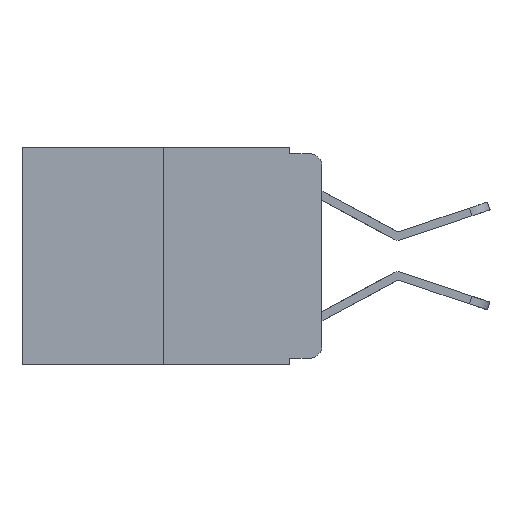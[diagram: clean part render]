
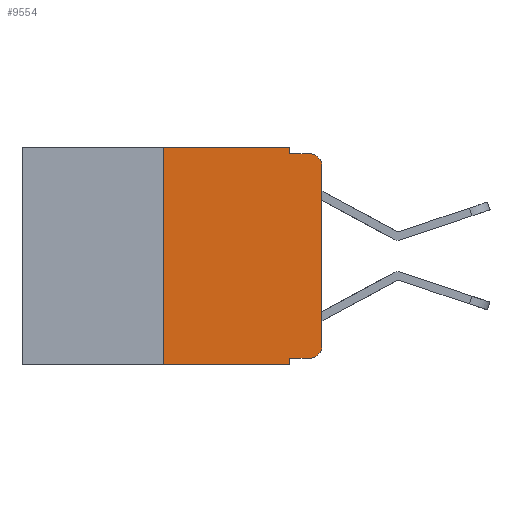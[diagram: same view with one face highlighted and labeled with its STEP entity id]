
A CAD part, left-side view. The second image highlights one B-rep face of the part: STEP entity #9554.
In plain terms, the highlighted planar face has unit normal (-1, 0, 0).
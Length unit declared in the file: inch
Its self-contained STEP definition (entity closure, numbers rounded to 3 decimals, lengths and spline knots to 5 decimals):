
#33 = CARTESIAN_POINT ( 'NONE',  ( 0., 0.473, 0. ) ) ;
#319 = CARTESIAN_POINT ( 'NONE',  ( 0., 0., 0. ) ) ;
#539 = DIRECTION ( 'NONE',  ( -1., 0., 0. ) ) ;
#790 = VECTOR ( 'NONE', #9614, 39.37008 ) ;
#947 = LINE ( 'NONE', #33, #13741 ) ;
#1215 = LINE ( 'NONE', #3589, #790 ) ;
#1332 = FACE_OUTER_BOUND ( 'NONE', #8569, .T. ) ;
#1608 = VERTEX_POINT ( 'NONE', #3708 ) ;
#1695 = ORIENTED_EDGE ( 'NONE', *, *, #7342, .F. ) ;
#1735 = AXIS2_PLACEMENT_3D ( 'NONE', #8056, #539, #9251 ) ;
#2065 = LINE ( 'NONE', #319, #2474 ) ;
#2474 = VECTOR ( 'NONE', #9069, 39.37008 ) ;
#2767 = DIRECTION ( 'NONE',  ( 0., -1., 0. ) ) ;
#2843 = DIRECTION ( 'NONE',  ( 0., -1., 0. ) ) ;
#2964 = ORIENTED_EDGE ( 'NONE', *, *, #14952, .T. ) ;
#3030 = VERTEX_POINT ( 'NONE', #7728 ) ;
#3143 = ORIENTED_EDGE ( 'NONE', *, *, #15994, .F. ) ;
#3589 = CARTESIAN_POINT ( 'NONE',  ( 0., 0.051, 0. ) ) ;
#3666 = PLANE ( 'NONE',  #10680 ) ;
#3708 = CARTESIAN_POINT ( 'NONE',  ( 0., 0., -0.03 ) ) ;
#3801 = ORIENTED_EDGE ( 'NONE', *, *, #5051, .F. ) ;
#4119 = DIRECTION ( 'NONE',  ( 0., -1., 0. ) ) ;
#4185 = DIRECTION ( 'NONE',  ( 0., 0., 1. ) ) ;
#4204 = VERTEX_POINT ( 'NONE', #11322 ) ;
#4241 = VERTEX_POINT ( 'NONE', #11829 ) ;
#4921 = DIRECTION ( 'NONE',  ( 0., 0., -1. ) ) ;
#4965 = ORIENTED_EDGE ( 'NONE', *, *, #9087, .T. ) ;
#5051 = EDGE_CURVE ( 'NONE', #4241, #13048, #6889, .T. ) ;
#5400 = VERTEX_POINT ( 'NONE', #9949 ) ;
#5528 = CARTESIAN_POINT ( 'NONE',  ( 0., 0., -0.313 ) ) ;
#6500 = CARTESIAN_POINT ( 'NONE',  ( 0., 0.02, -0.03 ) ) ;
#6889 = LINE ( 'NONE', #6901, #9726 ) ;
#6901 = CARTESIAN_POINT ( 'NONE',  ( 0., 0.051, 0. ) ) ;
#7060 = CARTESIAN_POINT ( 'NONE',  ( 0., 0.473, 0. ) ) ;
#7342 = EDGE_CURVE ( 'NONE', #4204, #11573, #947, .T. ) ;
#7368 = EDGE_CURVE ( 'NONE', #1608, #15202, #10515, .T. ) ;
#7493 = VERTEX_POINT ( 'NONE', #5528 ) ;
#7577 = VECTOR ( 'NONE', #12382, 39.37008 ) ;
#7620 = CARTESIAN_POINT ( 'NONE',  ( 0., 0.051, -0.01 ) ) ;
#7711 = DIRECTION ( 'NONE',  ( 0., 0., -1. ) ) ;
#7728 = CARTESIAN_POINT ( 'NONE',  ( 0., 0.25, -0.343 ) ) ;
#7968 = LINE ( 'NONE', #9928, #7577 ) ;
#8056 = CARTESIAN_POINT ( 'NONE',  ( 0., 0.02, -0.313 ) ) ;
#8528 = ORIENTED_EDGE ( 'NONE', *, *, #9886, .T. ) ;
#8569 = EDGE_LOOP ( 'NONE', ( #9623, #10857, #14451, #3143, #1695, #9246, #2964, #3801, #4965, #8528 ) ) ;
#8946 = CARTESIAN_POINT ( 'NONE',  ( 0., 0.051, -0.01 ) ) ;
#8979 = CARTESIAN_POINT ( 'NONE',  ( 0., 0.25, 0. ) ) ;
#9069 = DIRECTION ( 'NONE',  ( 0., 0., 1. ) ) ;
#9087 = EDGE_CURVE ( 'NONE', #4241, #5400, #7968, .T. ) ;
#9246 = ORIENTED_EDGE ( 'NONE', *, *, #12351, .F. ) ;
#9251 = DIRECTION ( 'NONE',  ( 0., 0., -1. ) ) ;
#9341 = VECTOR ( 'NONE', #4185, 39.37008 ) ;
#9554 = ADVANCED_FACE ( 'NONE', ( #1332 ), #3666, .F. ) ;
#9614 = DIRECTION ( 'NONE',  ( 0., 0., -1. ) ) ;
#9623 = ORIENTED_EDGE ( 'NONE', *, *, #15023, .T. ) ;
#9726 = VECTOR ( 'NONE', #15355, 39.37008 ) ;
#9732 = LINE ( 'NONE', #8979, #9341 ) ;
#9768 = VECTOR ( 'NONE', #4119, 39.37008 ) ;
#9886 = EDGE_CURVE ( 'NONE', #5400, #7493, #11627, .T. ) ;
#9928 = CARTESIAN_POINT ( 'NONE',  ( 0., 0.051, -0.333 ) ) ;
#9949 = CARTESIAN_POINT ( 'NONE',  ( 0., 0.02, -0.333 ) ) ;
#10515 = CIRCLE ( 'NONE', #12985, 0.02 ) ;
#10680 = AXIS2_PLACEMENT_3D ( 'NONE', #7060, #12224, #4921 ) ;
#10857 = ORIENTED_EDGE ( 'NONE', *, *, #7368, .T. ) ;
#11322 = CARTESIAN_POINT ( 'NONE',  ( 0., 0.25, 0. ) ) ;
#11573 = VERTEX_POINT ( 'NONE', #14997 ) ;
#11610 = EDGE_CURVE ( 'NONE', #15546, #15202, #15291, .T. ) ;
#11627 = CIRCLE ( 'NONE', #1735, 0.02 ) ;
#11829 = CARTESIAN_POINT ( 'NONE',  ( 0., 0.051, -0.333 ) ) ;
#11959 = CARTESIAN_POINT ( 'NONE',  ( 0., 0.02, -0.01 ) ) ;
#12224 = DIRECTION ( 'NONE',  ( 1., 0., 0. ) ) ;
#12351 = EDGE_CURVE ( 'NONE', #3030, #4204, #9732, .T. ) ;
#12382 = DIRECTION ( 'NONE',  ( 0., -1., 0. ) ) ;
#12644 = CARTESIAN_POINT ( 'NONE',  ( 0., 0.473, -0.343 ) ) ;
#12686 = LINE ( 'NONE', #12644, #9768 ) ;
#12985 = AXIS2_PLACEMENT_3D ( 'NONE', #6500, #15024, #7711 ) ;
#13048 = VERTEX_POINT ( 'NONE', #13974 ) ;
#13741 = VECTOR ( 'NONE', #2767, 39.37008 ) ;
#13974 = CARTESIAN_POINT ( 'NONE',  ( 0., 0.051, -0.343 ) ) ;
#14451 = ORIENTED_EDGE ( 'NONE', *, *, #11610, .F. ) ;
#14952 = EDGE_CURVE ( 'NONE', #3030, #13048, #12686, .T. ) ;
#14997 = CARTESIAN_POINT ( 'NONE',  ( 0., 0.051, 0. ) ) ;
#15023 = EDGE_CURVE ( 'NONE', #7493, #1608, #2065, .T. ) ;
#15024 = DIRECTION ( 'NONE',  ( -1., 0., 0. ) ) ;
#15202 = VERTEX_POINT ( 'NONE', #11959 ) ;
#15291 = LINE ( 'NONE', #8946, #15651 ) ;
#15355 = DIRECTION ( 'NONE',  ( 0., 0., -1. ) ) ;
#15546 = VERTEX_POINT ( 'NONE', #7620 ) ;
#15651 = VECTOR ( 'NONE', #2843, 39.37008 ) ;
#15994 = EDGE_CURVE ( 'NONE', #11573, #15546, #1215, .T. ) ;
